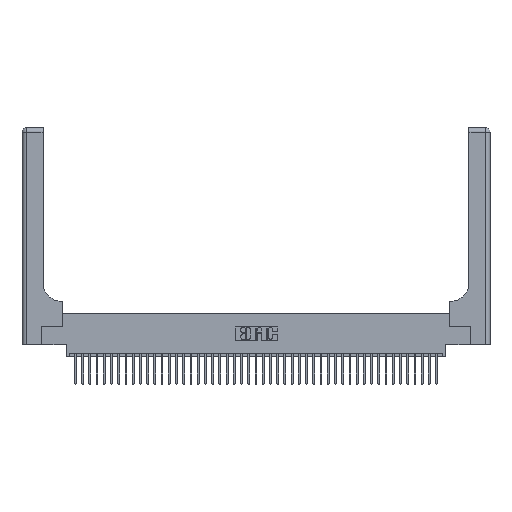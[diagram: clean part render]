
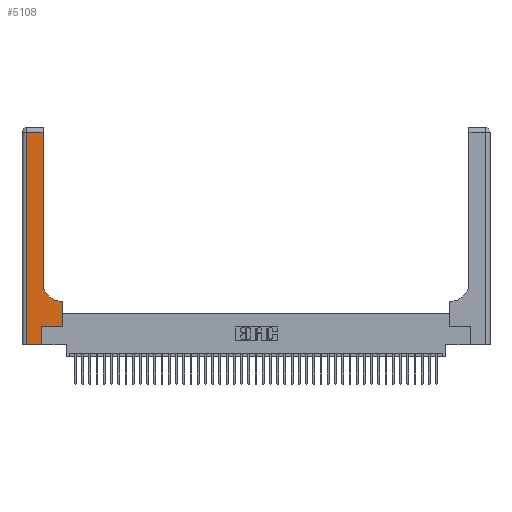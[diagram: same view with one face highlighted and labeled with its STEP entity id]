
A CAD part, top view. The second image highlights one B-rep face of the part: STEP entity #5108.
In plain terms, the highlighted planar face has unit normal (0, 0, 1).
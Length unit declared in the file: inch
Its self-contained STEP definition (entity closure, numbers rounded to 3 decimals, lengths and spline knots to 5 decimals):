
#820 = CARTESIAN_POINT ( 'NONE',  ( 0.269, 0., 0.37 ) ) ;
#1229 = CARTESIAN_POINT ( 'NONE',  ( 0.06, 3., 0.37 ) ) ;
#1907 = DIRECTION ( 'NONE',  ( 0., 0., -1. ) ) ;
#2093 = LINE ( 'NONE', #1229, #30324 ) ;
#2265 = LINE ( 'NONE', #22835, #37918 ) ;
#2437 = EDGE_CURVE ( 'NONE', #15924, #16219, #34579, .T. ) ;
#3513 = VERTEX_POINT ( 'NONE', #42865 ) ;
#3876 = CARTESIAN_POINT ( 'NONE',  ( 0.5415, 0.6, 0.37 ) ) ;
#4652 = VECTOR ( 'NONE', #27101, 39.37008 ) ;
#5108 = ADVANCED_FACE ( 'NONE', ( #27377 ), #11648, .F. ) ;
#6656 = EDGE_LOOP ( 'NONE', ( #32600, #16403, #11693, #43006, #26312, #12386, #31070, #34716, #44014 ) ) ;
#7467 = CARTESIAN_POINT ( 'NONE',  ( 0.5585, 0.6, 0.37 ) ) ;
#8041 = EDGE_CURVE ( 'NONE', #21790, #13928, #2265, .T. ) ;
#8142 = EDGE_CURVE ( 'NONE', #39938, #3513, #34217, .T. ) ;
#8461 = VECTOR ( 'NONE', #10683, 39.37008 ) ;
#10683 = DIRECTION ( 'NONE',  ( -1., 0., 0. ) ) ;
#10899 = EDGE_CURVE ( 'NONE', #37598, #40144, #13698, .T. ) ;
#11648 = PLANE ( 'NONE',  #22509 ) ;
#11693 = ORIENTED_EDGE ( 'NONE', *, *, #36518, .T. ) ;
#12386 = ORIENTED_EDGE ( 'NONE', *, *, #8142, .T. ) ;
#12670 = EDGE_CURVE ( 'NONE', #19834, #15924, #18072, .T. ) ;
#13131 = CARTESIAN_POINT ( 'NONE',  ( 0.2915, 0.85, 0.37 ) ) ;
#13698 = LINE ( 'NONE', #33838, #4652 ) ;
#13928 = VERTEX_POINT ( 'NONE', #3876 ) ;
#15086 = VECTOR ( 'NONE', #19749, 39.37008 ) ;
#15924 = VERTEX_POINT ( 'NONE', #31271 ) ;
#16080 = VECTOR ( 'NONE', #16581, 39.37008 ) ;
#16219 = VERTEX_POINT ( 'NONE', #32590 ) ;
#16330 = CARTESIAN_POINT ( 'NONE',  ( 0.5585, 0.25, 0.37 ) ) ;
#16403 = ORIENTED_EDGE ( 'NONE', *, *, #2437, .T. ) ;
#16570 = EDGE_CURVE ( 'NONE', #13928, #19834, #18779, .T. ) ;
#16581 = DIRECTION ( 'NONE',  ( 1., 0., 0. ) ) ;
#18072 = LINE ( 'NONE', #18939, #26078 ) ;
#18487 = DIRECTION ( 'NONE',  ( -1., 0., 0. ) ) ;
#18779 = CIRCLE ( 'NONE', #23306, 0.25 ) ;
#18939 = CARTESIAN_POINT ( 'NONE',  ( 0.2915, 3., 0.37 ) ) ;
#19749 = DIRECTION ( 'NONE',  ( 0., 1., 0. ) ) ;
#19834 = VERTEX_POINT ( 'NONE', #13131 ) ;
#20172 = CARTESIAN_POINT ( 'NONE',  ( 0.269, 0.25, 0.37 ) ) ;
#21790 = VERTEX_POINT ( 'NONE', #7467 ) ;
#22255 = CARTESIAN_POINT ( 'NONE',  ( 0.5415, 0.85, 0.37 ) ) ;
#22509 = AXIS2_PLACEMENT_3D ( 'NONE', #35515, #38959, #18487 ) ;
#22835 = CARTESIAN_POINT ( 'NONE',  ( 0.2915, 0.6, 0.37 ) ) ;
#23280 = CARTESIAN_POINT ( 'NONE',  ( 0.269, 0.25, 0.37 ) ) ;
#23306 = AXIS2_PLACEMENT_3D ( 'NONE', #22255, #1907, #25696 ) ;
#25030 = DIRECTION ( 'NONE',  ( 0., -1., 0. ) ) ;
#25696 = DIRECTION ( 'NONE',  ( 1., 0., 0. ) ) ;
#26078 = VECTOR ( 'NONE', #29216, 39.37008 ) ;
#26312 = ORIENTED_EDGE ( 'NONE', *, *, #31518, .T. ) ;
#27101 = DIRECTION ( 'NONE',  ( 1., 0., 0. ) ) ;
#27377 = FACE_OUTER_BOUND ( 'NONE', #6656, .T. ) ;
#28641 = VECTOR ( 'NONE', #38105, 39.37008 ) ;
#29216 = DIRECTION ( 'NONE',  ( 0., 1., 0. ) ) ;
#29550 = EDGE_CURVE ( 'NONE', #3513, #21790, #33245, .T. ) ;
#29702 = DIRECTION ( 'NONE',  ( -1., 0., 0. ) ) ;
#29713 = LINE ( 'NONE', #34650, #28641 ) ;
#30324 = VECTOR ( 'NONE', #25030, 39.37008 ) ;
#30513 = CARTESIAN_POINT ( 'NONE',  ( 0.06, 0., 0.37 ) ) ;
#31070 = ORIENTED_EDGE ( 'NONE', *, *, #29550, .T. ) ;
#31115 = CARTESIAN_POINT ( 'NONE',  ( 0., 2.94, 0.37 ) ) ;
#31271 = CARTESIAN_POINT ( 'NONE',  ( 0.2915, 2.94, 0.37 ) ) ;
#31518 = EDGE_CURVE ( 'NONE', #40144, #39938, #29713, .T. ) ;
#32590 = CARTESIAN_POINT ( 'NONE',  ( 0.06, 2.94, 0.37 ) ) ;
#32600 = ORIENTED_EDGE ( 'NONE', *, *, #12670, .T. ) ;
#33245 = LINE ( 'NONE', #16330, #15086 ) ;
#33838 = CARTESIAN_POINT ( 'NONE',  ( 0., 0., 0.37 ) ) ;
#34217 = LINE ( 'NONE', #23280, #16080 ) ;
#34579 = LINE ( 'NONE', #31115, #8461 ) ;
#34650 = CARTESIAN_POINT ( 'NONE',  ( 0.269, 0., 0.37 ) ) ;
#34716 = ORIENTED_EDGE ( 'NONE', *, *, #8041, .T. ) ;
#35515 = CARTESIAN_POINT ( 'NONE',  ( 0., 3., 0.37 ) ) ;
#36518 = EDGE_CURVE ( 'NONE', #16219, #37598, #2093, .T. ) ;
#37598 = VERTEX_POINT ( 'NONE', #30513 ) ;
#37918 = VECTOR ( 'NONE', #29702, 39.37008 ) ;
#38105 = DIRECTION ( 'NONE',  ( 0., 1., 0. ) ) ;
#38959 = DIRECTION ( 'NONE',  ( 0., 0., -1. ) ) ;
#39938 = VERTEX_POINT ( 'NONE', #20172 ) ;
#40144 = VERTEX_POINT ( 'NONE', #820 ) ;
#42865 = CARTESIAN_POINT ( 'NONE',  ( 0.5585, 0.25, 0.37 ) ) ;
#43006 = ORIENTED_EDGE ( 'NONE', *, *, #10899, .T. ) ;
#44014 = ORIENTED_EDGE ( 'NONE', *, *, #16570, .T. ) ;
